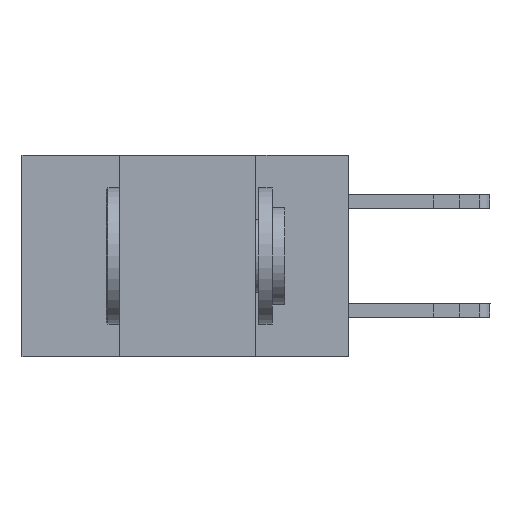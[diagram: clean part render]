
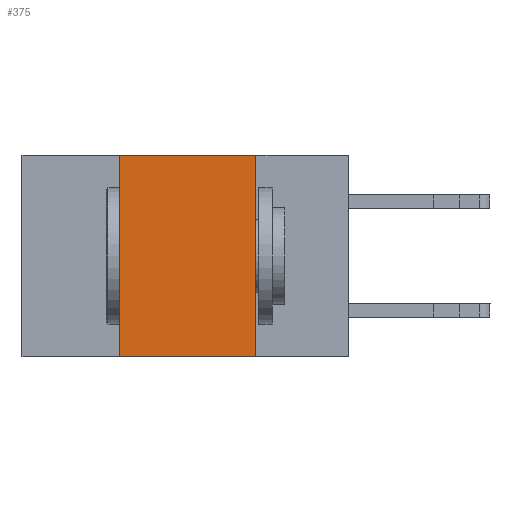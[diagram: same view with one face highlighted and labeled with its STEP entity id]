
A CAD part, left-side view. The second image highlights one B-rep face of the part: STEP entity #375.
In plain terms, the highlighted planar face has unit normal (-1, 0, 0).
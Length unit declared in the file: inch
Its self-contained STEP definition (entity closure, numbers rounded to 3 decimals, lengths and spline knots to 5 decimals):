
#375 = ADVANCED_FACE ( 'NONE', ( #14783 ), #13396, .F. ) ;
#901 = VECTOR ( 'NONE', #9487, 39.37008 ) ;
#1861 = CARTESIAN_POINT ( 'NONE',  ( 0., 0.6, 0. ) ) ;
#2407 = VERTEX_POINT ( 'NONE', #8936 ) ;
#4131 = EDGE_CURVE ( 'NONE', #4363, #10423, #13893, .T. ) ;
#4363 = VERTEX_POINT ( 'NONE', #9384 ) ;
#4616 = DIRECTION ( 'NONE',  ( 0., 0., -1. ) ) ;
#4806 = CARTESIAN_POINT ( 'NONE',  ( 0., 0.6, -0.37 ) ) ;
#5108 = LINE ( 'NONE', #6255, #901 ) ;
#5673 = ORIENTED_EDGE ( 'NONE', *, *, #8557, .F. ) ;
#5733 = VERTEX_POINT ( 'NONE', #11609 ) ;
#6173 = VECTOR ( 'NONE', #14957, 39.37008 ) ;
#6255 = CARTESIAN_POINT ( 'NONE',  ( 0., 0.42, -0.37 ) ) ;
#6690 = LINE ( 'NONE', #10175, #6173 ) ;
#7414 = CARTESIAN_POINT ( 'NONE',  ( 0., 0.17, -0.37 ) ) ;
#8557 = EDGE_CURVE ( 'NONE', #5733, #2407, #5108, .T. ) ;
#8936 = CARTESIAN_POINT ( 'NONE',  ( 0., 0.42, 0. ) ) ;
#9384 = CARTESIAN_POINT ( 'NONE',  ( 0., 0.17, 0. ) ) ;
#9487 = DIRECTION ( 'NONE',  ( 0., 0., 1. ) ) ;
#9657 = DIRECTION ( 'NONE',  ( 0., -1., 0. ) ) ;
#10175 = CARTESIAN_POINT ( 'NONE',  ( 0., 0.6, 0. ) ) ;
#10229 = LINE ( 'NONE', #4806, #13923 ) ;
#10423 = VERTEX_POINT ( 'NONE', #7414 ) ;
#11609 = CARTESIAN_POINT ( 'NONE',  ( 0., 0.42, -0.37 ) ) ;
#11612 = DIRECTION ( 'NONE',  ( 1., 0., 0. ) ) ;
#12310 = EDGE_LOOP ( 'NONE', ( #12417, #18852, #5673, #13649 ) ) ;
#12417 = ORIENTED_EDGE ( 'NONE', *, *, #4131, .F. ) ;
#13396 = PLANE ( 'NONE',  #20432 ) ;
#13407 = VECTOR ( 'NONE', #15416, 39.37008 ) ;
#13643 = EDGE_CURVE ( 'NONE', #5733, #10423, #10229, .T. ) ;
#13649 = ORIENTED_EDGE ( 'NONE', *, *, #13643, .T. ) ;
#13893 = LINE ( 'NONE', #14634, #13407 ) ;
#13923 = VECTOR ( 'NONE', #9657, 39.37008 ) ;
#14634 = CARTESIAN_POINT ( 'NONE',  ( 0., 0.17, -0.37 ) ) ;
#14783 = FACE_OUTER_BOUND ( 'NONE', #12310, .T. ) ;
#14957 = DIRECTION ( 'NONE',  ( 0., -1., 0. ) ) ;
#15416 = DIRECTION ( 'NONE',  ( 0., 0., -1. ) ) ;
#18852 = ORIENTED_EDGE ( 'NONE', *, *, #18898, .F. ) ;
#18898 = EDGE_CURVE ( 'NONE', #2407, #4363, #6690, .T. ) ;
#20432 = AXIS2_PLACEMENT_3D ( 'NONE', #1861, #11612, #4616 ) ;
